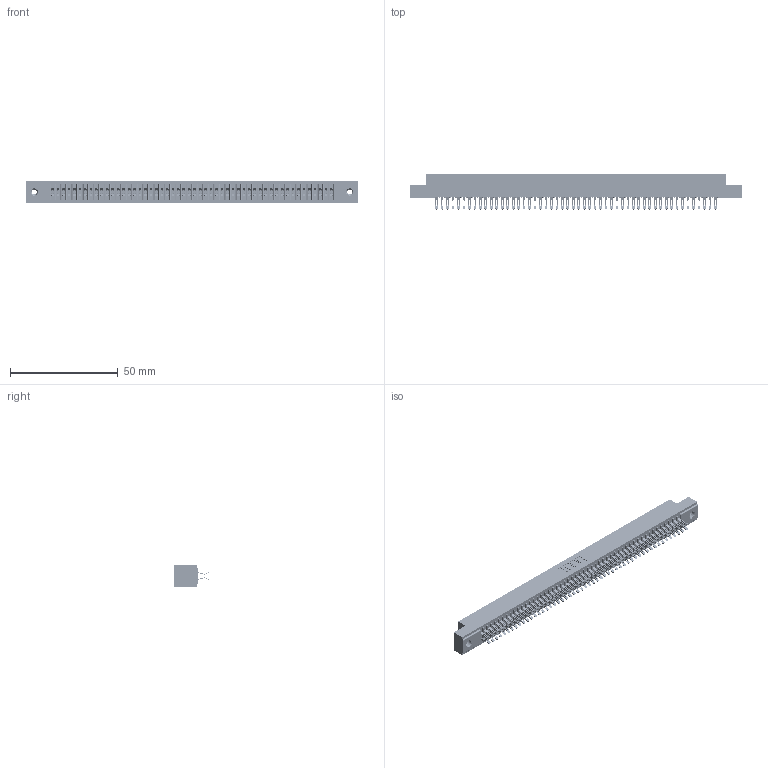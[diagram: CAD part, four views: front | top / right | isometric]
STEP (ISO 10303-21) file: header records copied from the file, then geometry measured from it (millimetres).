
FILE_DESCRIPTION (( 'STEP AP203' ), '1' );
FILE_NAME ('341-104-555-208.STEP', '2018-08-08T11:39:32', ( '' ), ( '' ), 'SwSTEP 2.0', 'SolidWorks 2016', '' );
FILE_SCHEMA (( 'CONFIG_CONTROL_DESIGN' ));
Length unit declared in the file: inch
Products named in the file (4): 341 Part_.156 (3.96) Dia Mounting Holes; 341-292-001_341-292-155; 345-250-001_345-250-003-102; 341-104-555-208
Assembly tree (107 placements, depth 2):
  341-104-555-208
    341 Part_.156 (3.96) Dia Mounting Holes
    341-292-001_341-292-155  x104
    345-250-001_345-250-003-102  x2
Bounding box: 154.31 x 16.31 x 10.16 mm (x, y, z)
Volume: 11529.1 mm3; surface area: 21648.9 mm2
Topology: 107 solids, 107 shells, 8288 faces, 24736 edges, 16098 vertices
Faces by surface type: plane 4468, cylinder 3596, sphere 106, torus 106, cone 12
Entity records: 63254 total; most frequent: CARTESIAN_POINT 10513, ORIENTED_EDGE 10432, DIRECTION 10196, EDGE_CURVE 5216, LINE 4206, VECTOR 4206, VERTEX_POINT 3296, AXIS2_PLACEMENT_3D 2995
